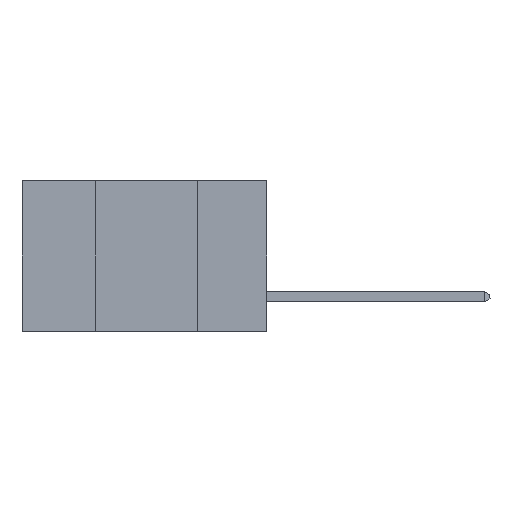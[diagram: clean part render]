
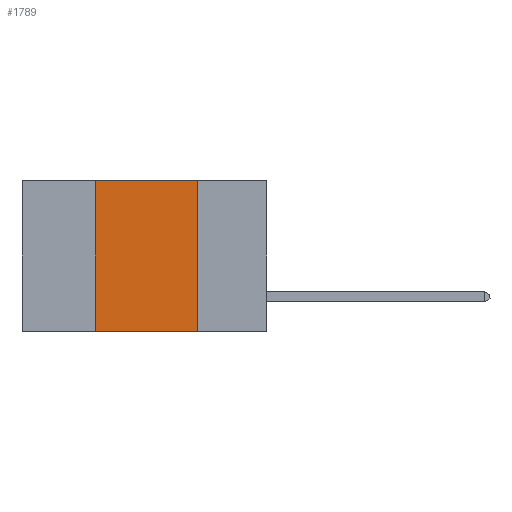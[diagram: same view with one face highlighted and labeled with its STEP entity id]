
A CAD part, left-side view. The second image highlights one B-rep face of the part: STEP entity #1789.
In plain terms, the highlighted planar face has unit normal (-1, 0, 0).
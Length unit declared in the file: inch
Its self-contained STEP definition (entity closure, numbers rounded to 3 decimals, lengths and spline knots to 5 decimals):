
#10 = CARTESIAN_POINT ( 'NONE',  ( 0., 0.6, -0.37 ) ) ;
#68 = ORIENTED_EDGE ( 'NONE', *, *, #2872, .F. ) ;
#378 = DIRECTION ( 'NONE',  ( 0., -1., 0. ) ) ;
#1005 = CARTESIAN_POINT ( 'NONE',  ( 0., 0.17, -0.37 ) ) ;
#1156 = VERTEX_POINT ( 'NONE', #8376 ) ;
#1533 = AXIS2_PLACEMENT_3D ( 'NONE', #2001, #7095, #6759 ) ;
#1789 = ADVANCED_FACE ( 'NONE', ( #6683 ), #5286, .F. ) ;
#1823 = VECTOR ( 'NONE', #8024, 39.37008 ) ;
#2001 = CARTESIAN_POINT ( 'NONE',  ( 0., 0.6, 0. ) ) ;
#2576 = EDGE_CURVE ( 'NONE', #6315, #5058, #3424, .T. ) ;
#2844 = VECTOR ( 'NONE', #378, 39.37008 ) ;
#2872 = EDGE_CURVE ( 'NONE', #1156, #6726, #4099, .T. ) ;
#3424 = LINE ( 'NONE', #10, #6880 ) ;
#3561 = CARTESIAN_POINT ( 'NONE',  ( 0., 0.42, 0. ) ) ;
#3729 = LINE ( 'NONE', #3561, #1823 ) ;
#4099 = LINE ( 'NONE', #9193, #2844 ) ;
#5058 = VERTEX_POINT ( 'NONE', #1005 ) ;
#5211 = DIRECTION ( 'NONE',  ( 0., 0., -1. ) ) ;
#5286 = PLANE ( 'NONE',  #1533 ) ;
#5513 = EDGE_CURVE ( 'NONE', #6726, #5058, #5960, .T. ) ;
#5763 = ORIENTED_EDGE ( 'NONE', *, *, #5513, .F. ) ;
#5960 = LINE ( 'NONE', #8157, #7011 ) ;
#6263 = EDGE_LOOP ( 'NONE', ( #5763, #68, #7089, #6952 ) ) ;
#6315 = VERTEX_POINT ( 'NONE', #8931 ) ;
#6602 = DIRECTION ( 'NONE',  ( 0., -1., 0. ) ) ;
#6683 = FACE_OUTER_BOUND ( 'NONE', #6263, .T. ) ;
#6718 = CARTESIAN_POINT ( 'NONE',  ( 0., 0.17, 0. ) ) ;
#6726 = VERTEX_POINT ( 'NONE', #6718 ) ;
#6759 = DIRECTION ( 'NONE',  ( 0., 0., -1. ) ) ;
#6880 = VECTOR ( 'NONE', #6602, 39.37008 ) ;
#6885 = EDGE_CURVE ( 'NONE', #6315, #1156, #3729, .T. ) ;
#6952 = ORIENTED_EDGE ( 'NONE', *, *, #2576, .T. ) ;
#7011 = VECTOR ( 'NONE', #5211, 39.37008 ) ;
#7089 = ORIENTED_EDGE ( 'NONE', *, *, #6885, .F. ) ;
#7095 = DIRECTION ( 'NONE',  ( 1., 0., 0. ) ) ;
#8024 = DIRECTION ( 'NONE',  ( 0., 0., 1. ) ) ;
#8157 = CARTESIAN_POINT ( 'NONE',  ( 0., 0.17, 0. ) ) ;
#8376 = CARTESIAN_POINT ( 'NONE',  ( 0., 0.42, 0. ) ) ;
#8931 = CARTESIAN_POINT ( 'NONE',  ( 0., 0.42, -0.37 ) ) ;
#9193 = CARTESIAN_POINT ( 'NONE',  ( 0., 0.6, 0. ) ) ;
